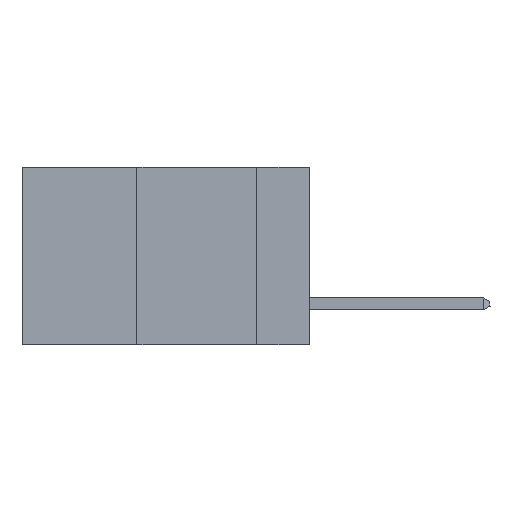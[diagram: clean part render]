
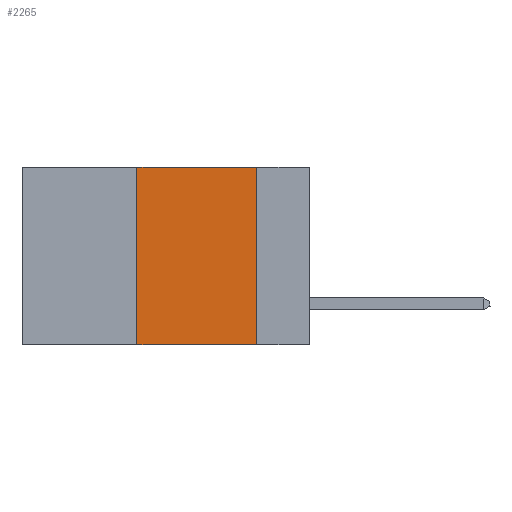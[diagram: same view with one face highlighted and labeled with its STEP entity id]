
A CAD part, left-side view. The second image highlights one B-rep face of the part: STEP entity #2265.
In plain terms, the highlighted planar face has unit normal (-1, 0, 0).
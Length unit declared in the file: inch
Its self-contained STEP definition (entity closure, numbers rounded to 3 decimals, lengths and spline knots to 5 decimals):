
#598 = ORIENTED_EDGE ( 'NONE', *, *, #17978, .F. ) ;
#2265 = ADVANCED_FACE ( 'NONE', ( #10161 ), #24560, .F. ) ;
#3782 = VERTEX_POINT ( 'NONE', #7202 ) ;
#3893 = LINE ( 'NONE', #14497, #23609 ) ;
#4602 = DIRECTION ( 'NONE',  ( 0., -1., 0. ) ) ;
#5118 = DIRECTION ( 'NONE',  ( 0., 0., -1. ) ) ;
#6186 = VERTEX_POINT ( 'NONE', #19836 ) ;
#6883 = CARTESIAN_POINT ( 'NONE',  ( 0., 0.36, 0. ) ) ;
#7202 = CARTESIAN_POINT ( 'NONE',  ( 0., 0.11, 0. ) ) ;
#9532 = VERTEX_POINT ( 'NONE', #24048 ) ;
#10161 = FACE_OUTER_BOUND ( 'NONE', #11415, .T. ) ;
#10858 = VERTEX_POINT ( 'NONE', #18424 ) ;
#11046 = CARTESIAN_POINT ( 'NONE',  ( 0., 0.6, 0. ) ) ;
#11415 = EDGE_LOOP ( 'NONE', ( #11482, #23067, #598, #25555 ) ) ;
#11482 = ORIENTED_EDGE ( 'NONE', *, *, #14655, .F. ) ;
#12589 = CARTESIAN_POINT ( 'NONE',  ( 0., 0.6, -0.37 ) ) ;
#12622 = DIRECTION ( 'NONE',  ( 0., -1., 0. ) ) ;
#14497 = CARTESIAN_POINT ( 'NONE',  ( 0., 0.6, 0. ) ) ;
#14655 = EDGE_CURVE ( 'NONE', #3782, #10858, #17594, .T. ) ;
#14945 = VECTOR ( 'NONE', #22615, 39.37008 ) ;
#17594 = LINE ( 'NONE', #21841, #23300 ) ;
#17978 = EDGE_CURVE ( 'NONE', #9532, #6186, #20215, .T. ) ;
#18424 = CARTESIAN_POINT ( 'NONE',  ( 0., 0.11, -0.37 ) ) ;
#19446 = VECTOR ( 'NONE', #4602, 39.37008 ) ;
#19836 = CARTESIAN_POINT ( 'NONE',  ( 0., 0.36, 0. ) ) ;
#20215 = LINE ( 'NONE', #6883, #14945 ) ;
#20361 = EDGE_CURVE ( 'NONE', #6186, #3782, #3893, .T. ) ;
#21841 = CARTESIAN_POINT ( 'NONE',  ( 0., 0.11, 0. ) ) ;
#22615 = DIRECTION ( 'NONE',  ( 0., 0., 1. ) ) ;
#23067 = ORIENTED_EDGE ( 'NONE', *, *, #20361, .F. ) ;
#23300 = VECTOR ( 'NONE', #25544, 39.37008 ) ;
#23609 = VECTOR ( 'NONE', #12622, 39.37008 ) ;
#24048 = CARTESIAN_POINT ( 'NONE',  ( 0., 0.36, -0.37 ) ) ;
#24451 = LINE ( 'NONE', #12589, #19446 ) ;
#24560 = PLANE ( 'NONE',  #25476 ) ;
#25099 = DIRECTION ( 'NONE',  ( 1., 0., 0. ) ) ;
#25271 = EDGE_CURVE ( 'NONE', #9532, #10858, #24451, .T. ) ;
#25476 = AXIS2_PLACEMENT_3D ( 'NONE', #11046, #25099, #5118 ) ;
#25544 = DIRECTION ( 'NONE',  ( 0., 0., -1. ) ) ;
#25555 = ORIENTED_EDGE ( 'NONE', *, *, #25271, .T. ) ;
